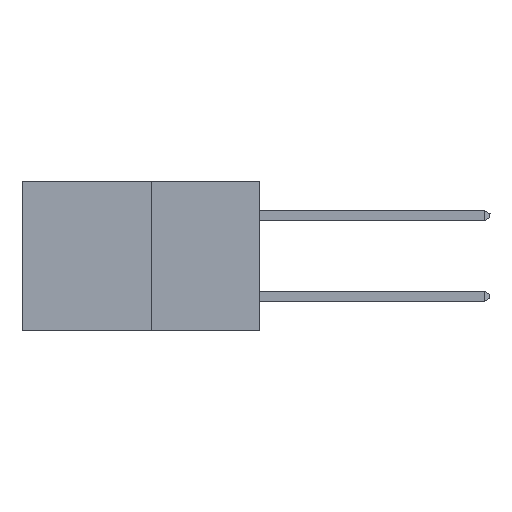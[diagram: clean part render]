
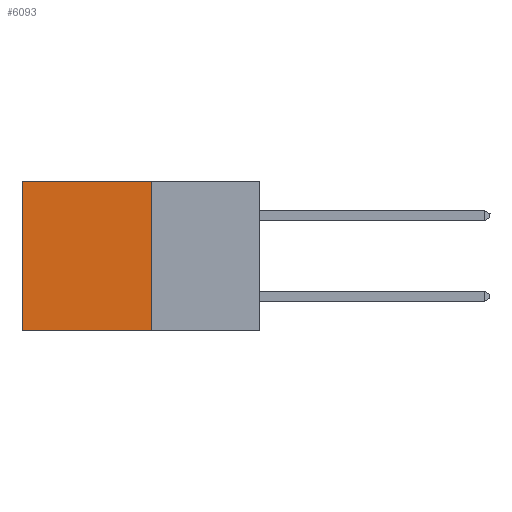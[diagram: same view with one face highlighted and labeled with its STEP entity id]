
A CAD part, left-side view. The second image highlights one B-rep face of the part: STEP entity #6093.
In plain terms, the highlighted planar face has unit normal (-1, 0, 0).
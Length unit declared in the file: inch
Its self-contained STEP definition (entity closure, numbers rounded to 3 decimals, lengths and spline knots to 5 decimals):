
#245 = EDGE_CURVE ( 'NONE', #5284, #10261, #11072, .T. ) ;
#363 = VERTEX_POINT ( 'NONE', #4726 ) ;
#368 = CARTESIAN_POINT ( 'NONE',  ( 0.277, 0.59, 0. ) ) ;
#469 = LINE ( 'NONE', #6528, #9499 ) ;
#654 = CARTESIAN_POINT ( 'NONE',  ( 0.277, 0.27, -0.37 ) ) ;
#1177 = DIRECTION ( 'NONE',  ( 0., 0., -1. ) ) ;
#1677 = EDGE_CURVE ( 'NONE', #363, #10261, #1948, .T. ) ;
#1948 = LINE ( 'NONE', #2346, #10795 ) ;
#2332 = DIRECTION ( 'NONE',  ( 0., 1., 0. ) ) ;
#2346 = CARTESIAN_POINT ( 'NONE',  ( 0.277, 0.27, -0.37 ) ) ;
#2464 = VERTEX_POINT ( 'NONE', #9216 ) ;
#2503 = DIRECTION ( 'NONE',  ( 1., 0., 0. ) ) ;
#2945 = EDGE_LOOP ( 'NONE', ( #8067, #7644, #9128, #10464 ) ) ;
#4029 = CARTESIAN_POINT ( 'NONE',  ( 0.277, 0.27, 0. ) ) ;
#4599 = CARTESIAN_POINT ( 'NONE',  ( 0.277, 0.59, -0.37 ) ) ;
#4726 = CARTESIAN_POINT ( 'NONE',  ( 0.277, 0.27, -0.37 ) ) ;
#4790 = CARTESIAN_POINT ( 'NONE',  ( 0.277, 0.59, -0.37 ) ) ;
#4872 = DIRECTION ( 'NONE',  ( 0., 0., -1. ) ) ;
#5284 = VERTEX_POINT ( 'NONE', #368 ) ;
#5333 = EDGE_CURVE ( 'NONE', #2464, #5284, #5376, .T. ) ;
#5376 = LINE ( 'NONE', #4029, #7851 ) ;
#6093 = ADVANCED_FACE ( 'NONE', ( #10790 ), #7748, .F. ) ;
#6528 = CARTESIAN_POINT ( 'NONE',  ( 0.277, 0.27, -0.37 ) ) ;
#6678 = DIRECTION ( 'NONE',  ( 0., 1., 0. ) ) ;
#7177 = AXIS2_PLACEMENT_3D ( 'NONE', #654, #2503, #8582 ) ;
#7644 = ORIENTED_EDGE ( 'NONE', *, *, #1677, .F. ) ;
#7748 = PLANE ( 'NONE',  #7177 ) ;
#7851 = VECTOR ( 'NONE', #6678, 39.37008 ) ;
#7952 = EDGE_CURVE ( 'NONE', #2464, #363, #469, .T. ) ;
#8067 = ORIENTED_EDGE ( 'NONE', *, *, #245, .T. ) ;
#8582 = DIRECTION ( 'NONE',  ( 0., 0., -1. ) ) ;
#9128 = ORIENTED_EDGE ( 'NONE', *, *, #7952, .F. ) ;
#9216 = CARTESIAN_POINT ( 'NONE',  ( 0.277, 0.27, 0. ) ) ;
#9499 = VECTOR ( 'NONE', #1177, 39.37008 ) ;
#10261 = VERTEX_POINT ( 'NONE', #4599 ) ;
#10464 = ORIENTED_EDGE ( 'NONE', *, *, #5333, .T. ) ;
#10790 = FACE_OUTER_BOUND ( 'NONE', #2945, .T. ) ;
#10795 = VECTOR ( 'NONE', #2332, 39.37008 ) ;
#10823 = VECTOR ( 'NONE', #4872, 39.37008 ) ;
#11072 = LINE ( 'NONE', #4790, #10823 ) ;
